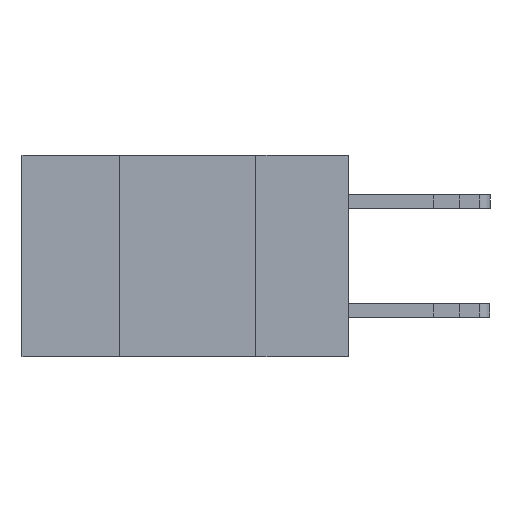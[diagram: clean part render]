
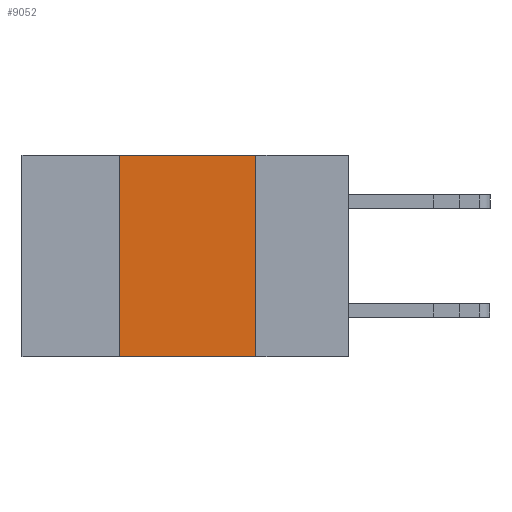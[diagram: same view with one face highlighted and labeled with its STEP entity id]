
A CAD part, left-side view. The second image highlights one B-rep face of the part: STEP entity #9052.
In plain terms, the highlighted planar face has unit normal (-1, 0, 0).
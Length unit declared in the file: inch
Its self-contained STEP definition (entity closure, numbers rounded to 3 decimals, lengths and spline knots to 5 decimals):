
#144 = DIRECTION ( 'NONE',  ( 0., 0., -1. ) ) ;
#824 = VECTOR ( 'NONE', #9280, 39.37008 ) ;
#894 = CARTESIAN_POINT ( 'NONE',  ( 0., 0.42, 0. ) ) ;
#963 = ORIENTED_EDGE ( 'NONE', *, *, #8304, .F. ) ;
#1087 = VERTEX_POINT ( 'NONE', #10902 ) ;
#1164 = EDGE_LOOP ( 'NONE', ( #4657, #963, #9484, #7635 ) ) ;
#1339 = VECTOR ( 'NONE', #6429, 39.37008 ) ;
#1988 = VERTEX_POINT ( 'NONE', #894 ) ;
#3123 = DIRECTION ( 'NONE',  ( 0., -1., 0. ) ) ;
#3669 = LINE ( 'NONE', #7327, #824 ) ;
#4395 = LINE ( 'NONE', #10680, #7103 ) ;
#4416 = PLANE ( 'NONE',  #5101 ) ;
#4657 = ORIENTED_EDGE ( 'NONE', *, *, #13116, .F. ) ;
#4741 = CARTESIAN_POINT ( 'NONE',  ( 0., 0.17, -0.37 ) ) ;
#5101 = AXIS2_PLACEMENT_3D ( 'NONE', #12333, #6472, #144 ) ;
#5792 = DIRECTION ( 'NONE',  ( 0., 0., 1. ) ) ;
#6429 = DIRECTION ( 'NONE',  ( 0., 0., -1. ) ) ;
#6472 = DIRECTION ( 'NONE',  ( 1., 0., 0. ) ) ;
#6640 = EDGE_CURVE ( 'NONE', #7263, #1988, #4395, .T. ) ;
#6653 = VERTEX_POINT ( 'NONE', #4741 ) ;
#7103 = VECTOR ( 'NONE', #5792, 39.37008 ) ;
#7263 = VERTEX_POINT ( 'NONE', #11566 ) ;
#7327 = CARTESIAN_POINT ( 'NONE',  ( 0., 0.6, 0. ) ) ;
#7601 = LINE ( 'NONE', #10164, #12482 ) ;
#7635 = ORIENTED_EDGE ( 'NONE', *, *, #9929, .T. ) ;
#8304 = EDGE_CURVE ( 'NONE', #1988, #1087, #3669, .T. ) ;
#9052 = ADVANCED_FACE ( 'NONE', ( #12211 ), #4416, .F. ) ;
#9280 = DIRECTION ( 'NONE',  ( 0., -1., 0. ) ) ;
#9484 = ORIENTED_EDGE ( 'NONE', *, *, #6640, .F. ) ;
#9532 = LINE ( 'NONE', #12286, #1339 ) ;
#9929 = EDGE_CURVE ( 'NONE', #7263, #6653, #7601, .T. ) ;
#10164 = CARTESIAN_POINT ( 'NONE',  ( 0., 0.6, -0.37 ) ) ;
#10680 = CARTESIAN_POINT ( 'NONE',  ( 0., 0.42, 0. ) ) ;
#10902 = CARTESIAN_POINT ( 'NONE',  ( 0., 0.17, 0. ) ) ;
#11566 = CARTESIAN_POINT ( 'NONE',  ( 0., 0.42, -0.37 ) ) ;
#12211 = FACE_OUTER_BOUND ( 'NONE', #1164, .T. ) ;
#12286 = CARTESIAN_POINT ( 'NONE',  ( 0., 0.17, 0. ) ) ;
#12333 = CARTESIAN_POINT ( 'NONE',  ( 0., 0.6, 0. ) ) ;
#12482 = VECTOR ( 'NONE', #3123, 39.37008 ) ;
#13116 = EDGE_CURVE ( 'NONE', #1087, #6653, #9532, .T. ) ;
